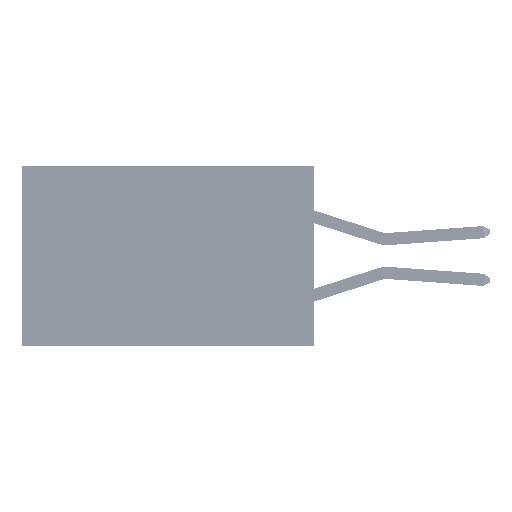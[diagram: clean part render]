
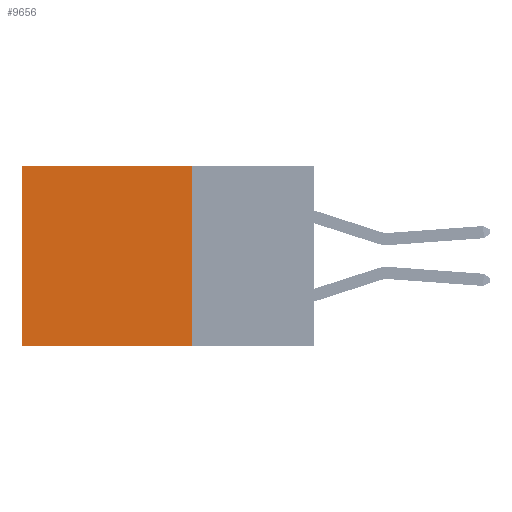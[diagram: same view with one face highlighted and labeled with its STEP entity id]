
A CAD part, left-side view. The second image highlights one B-rep face of the part: STEP entity #9656.
In plain terms, the highlighted planar face has unit normal (-1, 0, 0).
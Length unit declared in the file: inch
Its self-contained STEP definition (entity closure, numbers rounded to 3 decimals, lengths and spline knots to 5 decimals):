
#214 = CARTESIAN_POINT ( 'NONE',  ( 0.2875, 0.6, -0.37 ) ) ;
#611 = AXIS2_PLACEMENT_3D ( 'NONE', #26384, #2294, #22373 ) ;
#691 = VERTEX_POINT ( 'NONE', #14330 ) ;
#920 = LINE ( 'NONE', #36600, #43633 ) ;
#2294 = DIRECTION ( 'NONE',  ( 1., 0., 0. ) ) ;
#2336 = ORIENTED_EDGE ( 'NONE', *, *, #47123, .F. ) ;
#2476 = VERTEX_POINT ( 'NONE', #214 ) ;
#4218 = VECTOR ( 'NONE', #31166, 39.37008 ) ;
#5325 = DIRECTION ( 'NONE',  ( 0., 1., 0. ) ) ;
#5663 = CARTESIAN_POINT ( 'NONE',  ( 0.2875, 0.6, 0. ) ) ;
#9656 = ADVANCED_FACE ( 'NONE', ( #32564 ), #10278, .F. ) ;
#9856 = LINE ( 'NONE', #29040, #18482 ) ;
#10203 = ORIENTED_EDGE ( 'NONE', *, *, #27363, .T. ) ;
#10278 = PLANE ( 'NONE',  #611 ) ;
#13154 = CARTESIAN_POINT ( 'NONE',  ( 0.2875, 0.25, -0.37 ) ) ;
#14330 = CARTESIAN_POINT ( 'NONE',  ( 0.2875, 0.25, 0. ) ) ;
#14444 = LINE ( 'NONE', #24221, #30505 ) ;
#14577 = CARTESIAN_POINT ( 'NONE',  ( 0.2875, 0.25, 0. ) ) ;
#14689 = EDGE_CURVE ( 'NONE', #691, #19256, #9856, .T. ) ;
#18482 = VECTOR ( 'NONE', #5325, 39.37008 ) ;
#19256 = VERTEX_POINT ( 'NONE', #5663 ) ;
#22373 = DIRECTION ( 'NONE',  ( 0., 0., -1. ) ) ;
#24221 = CARTESIAN_POINT ( 'NONE',  ( 0.2875, 0.6, 0. ) ) ;
#26167 = EDGE_CURVE ( 'NONE', #50619, #2476, #920, .T. ) ;
#26384 = CARTESIAN_POINT ( 'NONE',  ( 0.2875, 0.25, 0. ) ) ;
#26696 = EDGE_LOOP ( 'NONE', ( #10203, #36601, #2336, #40335 ) ) ;
#27363 = EDGE_CURVE ( 'NONE', #19256, #2476, #14444, .T. ) ;
#29040 = CARTESIAN_POINT ( 'NONE',  ( 0.2875, 0.25, 0. ) ) ;
#30505 = VECTOR ( 'NONE', #35983, 39.37008 ) ;
#31166 = DIRECTION ( 'NONE',  ( 0., 0., -1. ) ) ;
#32564 = FACE_OUTER_BOUND ( 'NONE', #26696, .T. ) ;
#35983 = DIRECTION ( 'NONE',  ( 0., 0., -1. ) ) ;
#36600 = CARTESIAN_POINT ( 'NONE',  ( 0.2875, 0.25, -0.37 ) ) ;
#36601 = ORIENTED_EDGE ( 'NONE', *, *, #26167, .F. ) ;
#40335 = ORIENTED_EDGE ( 'NONE', *, *, #14689, .T. ) ;
#43633 = VECTOR ( 'NONE', #48230, 39.37008 ) ;
#45635 = LINE ( 'NONE', #14577, #4218 ) ;
#47123 = EDGE_CURVE ( 'NONE', #691, #50619, #45635, .T. ) ;
#48230 = DIRECTION ( 'NONE',  ( 0., 1., 0. ) ) ;
#50619 = VERTEX_POINT ( 'NONE', #13154 ) ;
